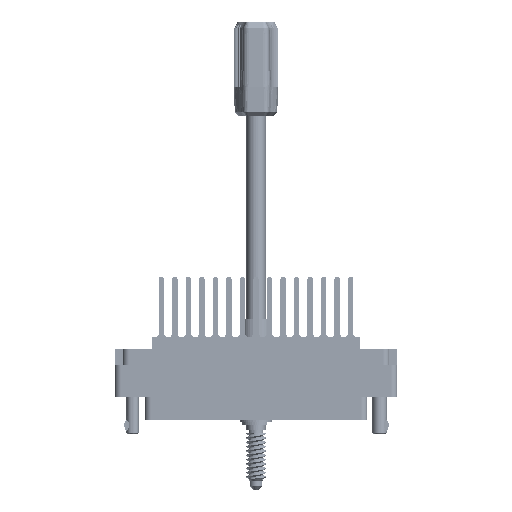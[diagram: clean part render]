
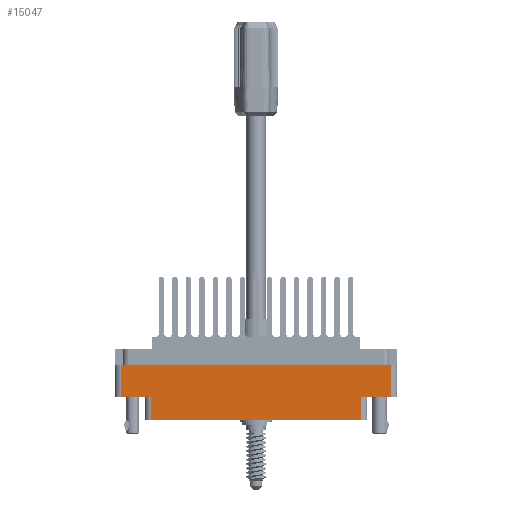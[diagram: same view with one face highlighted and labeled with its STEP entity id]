
A CAD part, front view. The second image highlights one B-rep face of the part: STEP entity #15047.
In plain terms, the highlighted planar face has unit normal (0, -1, 0).
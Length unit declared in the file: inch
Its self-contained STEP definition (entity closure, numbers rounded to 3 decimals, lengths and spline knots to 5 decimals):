
#1121 = DIRECTION ( 'NONE',  ( 0., 0., 1. ) ) ;
#1499 = LINE ( 'NONE', #60766, #27720 ) ;
#6118 = DIRECTION ( 'NONE',  ( 0., -1., 0. ) ) ;
#6536 = VECTOR ( 'NONE', #1121, 39.37008 ) ;
#8329 = FACE_OUTER_BOUND ( 'NONE', #16958, .T. ) ;
#9682 = VERTEX_POINT ( 'NONE', #57355 ) ;
#11586 = PLANE ( 'NONE',  #78979 ) ;
#11900 = CARTESIAN_POINT ( 'NONE',  ( 1.297, -0.617, -0.578 ) ) ;
#13412 = LINE ( 'NONE', #89210, #6536 ) ;
#13946 = EDGE_CURVE ( 'NONE', #80142, #30864, #38828, .T. ) ;
#15047 = ADVANCED_FACE ( 'NONE', ( #8329 ), #11586, .T. ) ;
#16958 = EDGE_LOOP ( 'NONE', ( #92510, #35620, #35250, #59866, #78295, #64831, #94104, #56932 ) ) ;
#18636 = EDGE_CURVE ( 'NONE', #80142, #36492, #42033, .T. ) ;
#18689 = CARTESIAN_POINT ( 'NONE',  ( -1.006, -0.617, -0.798 ) ) ;
#22121 = EDGE_CURVE ( 'NONE', #63433, #77131, #26683, .T. ) ;
#25347 = VECTOR ( 'NONE', #31669, 39.37008 ) ;
#26357 = DIRECTION ( 'NONE',  ( 0., 0., -1. ) ) ;
#26683 = LINE ( 'NONE', #72584, #39268 ) ;
#27720 = VECTOR ( 'NONE', #53056, 39.37008 ) ;
#27886 = EDGE_CURVE ( 'NONE', #71777, #63433, #86855, .T. ) ;
#29642 = VECTOR ( 'NONE', #78034, 39.37008 ) ;
#30864 = VERTEX_POINT ( 'NONE', #46365 ) ;
#31669 = DIRECTION ( 'NONE',  ( -1., 0., 0. ) ) ;
#32793 = CARTESIAN_POINT ( 'NONE',  ( -1.006, -0.617, -0.798 ) ) ;
#32851 = VECTOR ( 'NONE', #83984, 39.37008 ) ;
#33598 = CARTESIAN_POINT ( 'NONE',  ( 0., -0.617, -0.578 ) ) ;
#35250 = ORIENTED_EDGE ( 'NONE', *, *, #22121, .T. ) ;
#35620 = ORIENTED_EDGE ( 'NONE', *, *, #27886, .T. ) ;
#36492 = VERTEX_POINT ( 'NONE', #68926 ) ;
#38828 = LINE ( 'NONE', #64419, #56056 ) ;
#39268 = VECTOR ( 'NONE', #51506, 39.37008 ) ;
#39306 = EDGE_CURVE ( 'NONE', #49191, #9682, #47079, .T. ) ;
#40833 = CARTESIAN_POINT ( 'NONE',  ( 0., -0.617, -0.274 ) ) ;
#42033 = LINE ( 'NONE', #40833, #32851 ) ;
#43392 = LINE ( 'NONE', #33598, #29642 ) ;
#43864 = CARTESIAN_POINT ( 'NONE',  ( 0., -0.617, -0.578 ) ) ;
#45023 = DIRECTION ( 'NONE',  ( 0., 0., -1. ) ) ;
#46365 = CARTESIAN_POINT ( 'NONE',  ( -1.297, -0.617, -0.578 ) ) ;
#47079 = LINE ( 'NONE', #43864, #25347 ) ;
#49191 = VERTEX_POINT ( 'NONE', #11900 ) ;
#51332 = CARTESIAN_POINT ( 'NONE',  ( -1.297, -0.617, -0.274 ) ) ;
#51506 = DIRECTION ( 'NONE',  ( 1., 0., 0. ) ) ;
#53056 = DIRECTION ( 'NONE',  ( 0., 0., 1. ) ) ;
#53626 = CARTESIAN_POINT ( 'NONE',  ( -1.006, -0.617, -0.578 ) ) ;
#54248 = DIRECTION ( 'NONE',  ( 0., 0., -1. ) ) ;
#56056 = VECTOR ( 'NONE', #26357, 39.37008 ) ;
#56932 = ORIENTED_EDGE ( 'NONE', *, *, #13946, .T. ) ;
#57355 = CARTESIAN_POINT ( 'NONE',  ( 1.006, -0.617, -0.578 ) ) ;
#59866 = ORIENTED_EDGE ( 'NONE', *, *, #66965, .T. ) ;
#60766 = CARTESIAN_POINT ( 'NONE',  ( 1.006, -0.617, -0.578 ) ) ;
#61807 = EDGE_CURVE ( 'NONE', #30864, #71777, #43392, .T. ) ;
#63433 = VERTEX_POINT ( 'NONE', #18689 ) ;
#64419 = CARTESIAN_POINT ( 'NONE',  ( -1.297, -0.617, -0.798 ) ) ;
#64831 = ORIENTED_EDGE ( 'NONE', *, *, #78250, .T. ) ;
#66965 = EDGE_CURVE ( 'NONE', #77131, #9682, #1499, .T. ) ;
#68926 = CARTESIAN_POINT ( 'NONE',  ( 1.297, -0.617, -0.274 ) ) ;
#71777 = VERTEX_POINT ( 'NONE', #53626 ) ;
#72584 = CARTESIAN_POINT ( 'NONE',  ( -1.359, -0.617, -0.798 ) ) ;
#77131 = VERTEX_POINT ( 'NONE', #88266 ) ;
#77727 = VECTOR ( 'NONE', #54248, 39.37008 ) ;
#78034 = DIRECTION ( 'NONE',  ( 1., 0., 0. ) ) ;
#78250 = EDGE_CURVE ( 'NONE', #49191, #36492, #13412, .T. ) ;
#78295 = ORIENTED_EDGE ( 'NONE', *, *, #39306, .F. ) ;
#78962 = CARTESIAN_POINT ( 'NONE',  ( -1.359, -0.617, -0.798 ) ) ;
#78979 = AXIS2_PLACEMENT_3D ( 'NONE', #78962, #6118, #45023 ) ;
#80142 = VERTEX_POINT ( 'NONE', #51332 ) ;
#83984 = DIRECTION ( 'NONE',  ( 1., 0., 0. ) ) ;
#86855 = LINE ( 'NONE', #32793, #77727 ) ;
#88266 = CARTESIAN_POINT ( 'NONE',  ( 1.006, -0.617, -0.798 ) ) ;
#89210 = CARTESIAN_POINT ( 'NONE',  ( 1.297, -0.617, -0.798 ) ) ;
#92510 = ORIENTED_EDGE ( 'NONE', *, *, #61807, .T. ) ;
#94104 = ORIENTED_EDGE ( 'NONE', *, *, #18636, .F. ) ;
